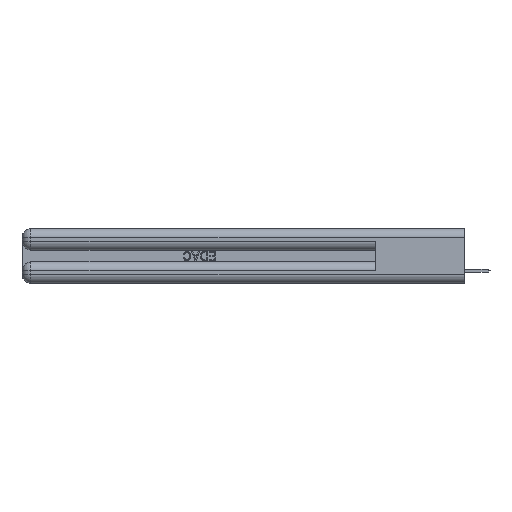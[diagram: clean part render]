
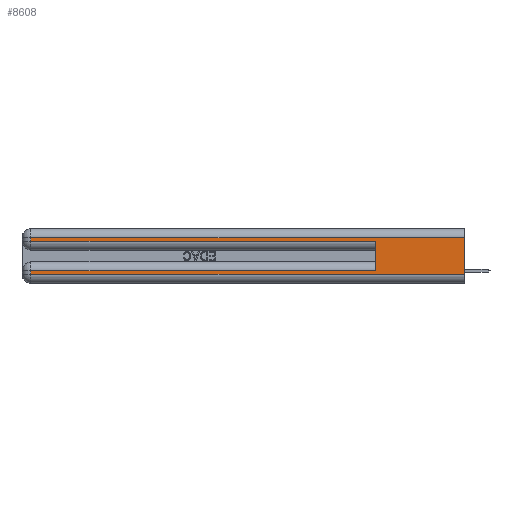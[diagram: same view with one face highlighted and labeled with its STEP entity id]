
A CAD part, left-side view. The second image highlights one B-rep face of the part: STEP entity #8608.
In plain terms, the highlighted planar face has unit normal (-1, 0, 0).
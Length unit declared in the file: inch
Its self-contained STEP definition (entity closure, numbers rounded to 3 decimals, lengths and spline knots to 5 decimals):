
#59 = LINE ( 'NONE', #38653, #42141 ) ;
#433 = LINE ( 'NONE', #32260, #25594 ) ;
#1530 = DIRECTION ( 'NONE',  ( 1., 0., 0. ) ) ;
#1792 = EDGE_CURVE ( 'NONE', #34693, #27654, #27838, .T. ) ;
#2082 = DIRECTION ( 'NONE',  ( 0., -1., 0. ) ) ;
#3311 = VECTOR ( 'NONE', #2082, 39.37008 ) ;
#3396 = LINE ( 'NONE', #12174, #36156 ) ;
#3672 = EDGE_CURVE ( 'NONE', #34693, #16288, #59, .T. ) ;
#4659 = CARTESIAN_POINT ( 'NONE',  ( 0., 2.94, 0.285 ) ) ;
#4808 = VECTOR ( 'NONE', #33678, 39.37008 ) ;
#5279 = EDGE_CURVE ( 'NONE', #22338, #16755, #433, .T. ) ;
#5923 = LINE ( 'NONE', #31987, #3311 ) ;
#5974 = VECTOR ( 'NONE', #12051, 39.37008 ) ;
#6172 = DIRECTION ( 'NONE',  ( 0., 0., -1. ) ) ;
#6854 = CARTESIAN_POINT ( 'NONE',  ( 0., 2.94, 0.37 ) ) ;
#7177 = CARTESIAN_POINT ( 'NONE',  ( 0., 2.94, 0.31 ) ) ;
#7574 = AXIS2_PLACEMENT_3D ( 'NONE', #24390, #1530, #6172 ) ;
#8608 = ADVANCED_FACE ( 'NONE', ( #13920 ), #21259, .F. ) ;
#9148 = CARTESIAN_POINT ( 'NONE',  ( 0., 2.94, 0.06 ) ) ;
#10800 = CARTESIAN_POINT ( 'NONE',  ( 0., 0.6, 0.145 ) ) ;
#12051 = DIRECTION ( 'NONE',  ( 0., 0., -1. ) ) ;
#12174 = CARTESIAN_POINT ( 'NONE',  ( 0., 0., 0.31 ) ) ;
#13264 = EDGE_CURVE ( 'NONE', #19144, #16755, #13639, .T. ) ;
#13349 = DIRECTION ( 'NONE',  ( 0., 1., 0. ) ) ;
#13639 = LINE ( 'NONE', #28793, #21345 ) ;
#13879 = CARTESIAN_POINT ( 'NONE',  ( 0., 0., 0.06 ) ) ;
#13920 = FACE_OUTER_BOUND ( 'NONE', #35461, .T. ) ;
#14070 = EDGE_CURVE ( 'NONE', #22338, #19840, #3396, .T. ) ;
#14888 = DIRECTION ( 'NONE',  ( 0., 1., 0. ) ) ;
#14904 = ORIENTED_EDGE ( 'NONE', *, *, #3672, .T. ) ;
#15900 = VERTEX_POINT ( 'NONE', #4659 ) ;
#16288 = VERTEX_POINT ( 'NONE', #21515 ) ;
#16755 = VERTEX_POINT ( 'NONE', #13879 ) ;
#16862 = CARTESIAN_POINT ( 'NONE',  ( 0., 0., 0.31 ) ) ;
#17311 = ORIENTED_EDGE ( 'NONE', *, *, #31415, .T. ) ;
#18285 = EDGE_CURVE ( 'NONE', #16288, #19144, #37702, .T. ) ;
#19144 = VERTEX_POINT ( 'NONE', #9148 ) ;
#19840 = VERTEX_POINT ( 'NONE', #7177 ) ;
#21259 = PLANE ( 'NONE',  #7574 ) ;
#21345 = VECTOR ( 'NONE', #28352, 39.37008 ) ;
#21515 = CARTESIAN_POINT ( 'NONE',  ( 0., 2.94, 0.085 ) ) ;
#22338 = VERTEX_POINT ( 'NONE', #16862 ) ;
#22854 = DIRECTION ( 'NONE',  ( 0., 0., -1. ) ) ;
#23523 = ORIENTED_EDGE ( 'NONE', *, *, #13264, .T. ) ;
#23953 = VECTOR ( 'NONE', #30111, 39.37008 ) ;
#24390 = CARTESIAN_POINT ( 'NONE',  ( 0., 0., 0.37 ) ) ;
#25594 = VECTOR ( 'NONE', #22854, 39.37008 ) ;
#27267 = CARTESIAN_POINT ( 'NONE',  ( 0., 0.6, 0.285 ) ) ;
#27654 = VERTEX_POINT ( 'NONE', #27267 ) ;
#27838 = LINE ( 'NONE', #10800, #4808 ) ;
#28352 = DIRECTION ( 'NONE',  ( 0., -1., 0. ) ) ;
#28793 = CARTESIAN_POINT ( 'NONE',  ( 0., 0., 0.06 ) ) ;
#30111 = DIRECTION ( 'NONE',  ( 0., 0., -1. ) ) ;
#31415 = EDGE_CURVE ( 'NONE', #15900, #27654, #5923, .T. ) ;
#31657 = CARTESIAN_POINT ( 'NONE',  ( 0., 2.94, 0.37 ) ) ;
#31987 = CARTESIAN_POINT ( 'NONE',  ( 0., 0., 0.285 ) ) ;
#32260 = CARTESIAN_POINT ( 'NONE',  ( 0., 0., 0.37 ) ) ;
#32407 = ORIENTED_EDGE ( 'NONE', *, *, #1792, .F. ) ;
#33663 = ORIENTED_EDGE ( 'NONE', *, *, #34834, .T. ) ;
#33678 = DIRECTION ( 'NONE',  ( 0., 0., 1. ) ) ;
#34693 = VERTEX_POINT ( 'NONE', #36203 ) ;
#34834 = EDGE_CURVE ( 'NONE', #19840, #15900, #38961, .T. ) ;
#35254 = ORIENTED_EDGE ( 'NONE', *, *, #18285, .T. ) ;
#35461 = EDGE_LOOP ( 'NONE', ( #38104, #41905, #33663, #17311, #32407, #14904, #35254, #23523 ) ) ;
#36156 = VECTOR ( 'NONE', #14888, 39.37008 ) ;
#36203 = CARTESIAN_POINT ( 'NONE',  ( 0., 0.6, 0.085 ) ) ;
#37702 = LINE ( 'NONE', #31657, #5974 ) ;
#38104 = ORIENTED_EDGE ( 'NONE', *, *, #5279, .F. ) ;
#38653 = CARTESIAN_POINT ( 'NONE',  ( 0., 0., 0.085 ) ) ;
#38961 = LINE ( 'NONE', #6854, #23953 ) ;
#41905 = ORIENTED_EDGE ( 'NONE', *, *, #14070, .T. ) ;
#42141 = VECTOR ( 'NONE', #13349, 39.37008 ) ;
